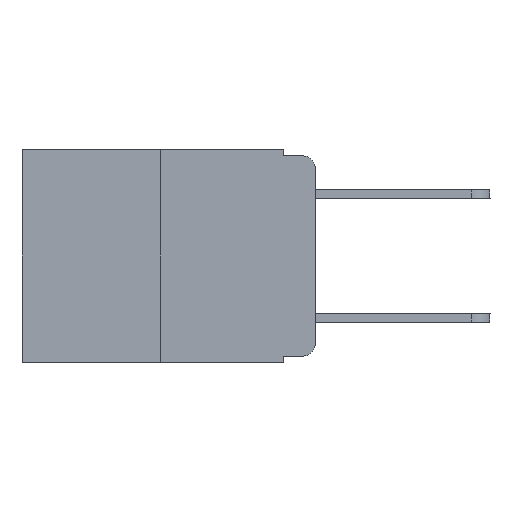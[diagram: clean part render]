
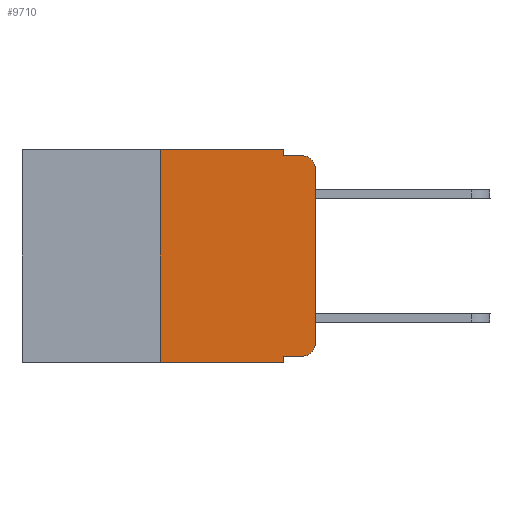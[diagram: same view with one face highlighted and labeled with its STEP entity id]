
A CAD part, left-side view. The second image highlights one B-rep face of the part: STEP entity #9710.
In plain terms, the highlighted planar face has unit normal (-1, 0, 0).
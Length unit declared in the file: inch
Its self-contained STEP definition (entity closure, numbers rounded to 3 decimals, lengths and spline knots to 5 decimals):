
#53 = CARTESIAN_POINT ( 'NONE',  ( 0., 0.02, -0.313 ) ) ;
#161 = VECTOR ( 'NONE', #4071, 39.37008 ) ;
#212 = DIRECTION ( 'NONE',  ( 1., 0., 0. ) ) ;
#253 = VECTOR ( 'NONE', #6656, 39.37008 ) ;
#276 = DIRECTION ( 'NONE',  ( 0., -1., 0. ) ) ;
#301 = ORIENTED_EDGE ( 'NONE', *, *, #6651, .F. ) ;
#363 = DIRECTION ( 'NONE',  ( 0., 0., 1. ) ) ;
#500 = CARTESIAN_POINT ( 'NONE',  ( 0., 0., 0. ) ) ;
#543 = EDGE_LOOP ( 'NONE', ( #8076, #6305, #7824, #6847, #2883, #301, #1526, #4783, #4809, #9727 ) ) ;
#1196 = EDGE_CURVE ( 'NONE', #5977, #3756, #8181, .T. ) ;
#1275 = CARTESIAN_POINT ( 'NONE',  ( 0., 0.25, -0.343 ) ) ;
#1448 = VECTOR ( 'NONE', #2631, 39.37008 ) ;
#1488 = VECTOR ( 'NONE', #363, 39.37008 ) ;
#1526 = ORIENTED_EDGE ( 'NONE', *, *, #3667, .T. ) ;
#1585 = CARTESIAN_POINT ( 'NONE',  ( 0., 0.051, -0.01 ) ) ;
#1654 = CARTESIAN_POINT ( 'NONE',  ( 0., 0.02, -0.333 ) ) ;
#1941 = VECTOR ( 'NONE', #3297, 39.37008 ) ;
#2204 = VECTOR ( 'NONE', #9762, 39.37008 ) ;
#2264 = LINE ( 'NONE', #6695, #253 ) ;
#2532 = CIRCLE ( 'NONE', #7644, 0.02 ) ;
#2631 = DIRECTION ( 'NONE',  ( 0., 0., 1. ) ) ;
#2684 = VERTEX_POINT ( 'NONE', #1654 ) ;
#2691 = CARTESIAN_POINT ( 'NONE',  ( 0., 0.02, -0.03 ) ) ;
#2705 = CARTESIAN_POINT ( 'NONE',  ( 0., 0.051, -0.01 ) ) ;
#2770 = VECTOR ( 'NONE', #276, 39.37008 ) ;
#2883 = ORIENTED_EDGE ( 'NONE', *, *, #5691, .F. ) ;
#3196 = CARTESIAN_POINT ( 'NONE',  ( 0., 0.473, -0.343 ) ) ;
#3252 = LINE ( 'NONE', #7106, #1488 ) ;
#3297 = DIRECTION ( 'NONE',  ( 0., 0., -1. ) ) ;
#3446 = VERTEX_POINT ( 'NONE', #4098 ) ;
#3496 = LINE ( 'NONE', #8485, #5391 ) ;
#3667 = EDGE_CURVE ( 'NONE', #3702, #3756, #6582, .T. ) ;
#3702 = VERTEX_POINT ( 'NONE', #1275 ) ;
#3756 = VERTEX_POINT ( 'NONE', #5948 ) ;
#3767 = VERTEX_POINT ( 'NONE', #5079 ) ;
#3789 = DIRECTION ( 'NONE',  ( 0., 0., -1. ) ) ;
#4066 = PLANE ( 'NONE',  #6803 ) ;
#4071 = DIRECTION ( 'NONE',  ( 0., -1., 0. ) ) ;
#4098 = CARTESIAN_POINT ( 'NONE',  ( 0., 0.02, -0.01 ) ) ;
#4783 = ORIENTED_EDGE ( 'NONE', *, *, #1196, .F. ) ;
#4801 = CARTESIAN_POINT ( 'NONE',  ( 0., 0.051, 0. ) ) ;
#4809 = ORIENTED_EDGE ( 'NONE', *, *, #5874, .T. ) ;
#5079 = CARTESIAN_POINT ( 'NONE',  ( 0., 0., -0.03 ) ) ;
#5333 = CARTESIAN_POINT ( 'NONE',  ( 0., 0.473, 0. ) ) ;
#5391 = VECTOR ( 'NONE', #6882, 39.37008 ) ;
#5424 = EDGE_CURVE ( 'NONE', #3767, #3446, #7389, .T. ) ;
#5447 = FACE_OUTER_BOUND ( 'NONE', #543, .T. ) ;
#5691 = EDGE_CURVE ( 'NONE', #7209, #9743, #6231, .T. ) ;
#5874 = EDGE_CURVE ( 'NONE', #5977, #2684, #3496, .T. ) ;
#5948 = CARTESIAN_POINT ( 'NONE',  ( 0., 0.051, -0.343 ) ) ;
#5977 = VERTEX_POINT ( 'NONE', #9309 ) ;
#6093 = LINE ( 'NONE', #1585, #161 ) ;
#6231 = LINE ( 'NONE', #5333, #2204 ) ;
#6305 = ORIENTED_EDGE ( 'NONE', *, *, #5424, .T. ) ;
#6357 = CARTESIAN_POINT ( 'NONE',  ( 0., 0.473, 0. ) ) ;
#6547 = LINE ( 'NONE', #500, #1448 ) ;
#6582 = LINE ( 'NONE', #3196, #2770 ) ;
#6651 = EDGE_CURVE ( 'NONE', #3702, #7209, #3252, .T. ) ;
#6656 = DIRECTION ( 'NONE',  ( 0., 0., -1. ) ) ;
#6695 = CARTESIAN_POINT ( 'NONE',  ( 0., 0.051, 0. ) ) ;
#6803 = AXIS2_PLACEMENT_3D ( 'NONE', #6357, #212, #7838 ) ;
#6847 = ORIENTED_EDGE ( 'NONE', *, *, #9526, .F. ) ;
#6882 = DIRECTION ( 'NONE',  ( 0., -1., 0. ) ) ;
#7013 = EDGE_CURVE ( 'NONE', #2684, #7725, #2532, .T. ) ;
#7106 = CARTESIAN_POINT ( 'NONE',  ( 0., 0.25, 0. ) ) ;
#7149 = AXIS2_PLACEMENT_3D ( 'NONE', #2691, #7948, #8750 ) ;
#7209 = VERTEX_POINT ( 'NONE', #8746 ) ;
#7389 = CIRCLE ( 'NONE', #7149, 0.02 ) ;
#7644 = AXIS2_PLACEMENT_3D ( 'NONE', #53, #9180, #3789 ) ;
#7677 = EDGE_CURVE ( 'NONE', #8072, #3446, #6093, .T. ) ;
#7725 = VERTEX_POINT ( 'NONE', #9167 ) ;
#7774 = CARTESIAN_POINT ( 'NONE',  ( 0., 0.051, 0. ) ) ;
#7824 = ORIENTED_EDGE ( 'NONE', *, *, #7677, .F. ) ;
#7838 = DIRECTION ( 'NONE',  ( 0., 0., -1. ) ) ;
#7948 = DIRECTION ( 'NONE',  ( -1., 0., 0. ) ) ;
#8067 = EDGE_CURVE ( 'NONE', #7725, #3767, #6547, .T. ) ;
#8072 = VERTEX_POINT ( 'NONE', #2705 ) ;
#8076 = ORIENTED_EDGE ( 'NONE', *, *, #8067, .T. ) ;
#8181 = LINE ( 'NONE', #7774, #1941 ) ;
#8485 = CARTESIAN_POINT ( 'NONE',  ( 0., 0.051, -0.333 ) ) ;
#8746 = CARTESIAN_POINT ( 'NONE',  ( 0., 0.25, 0. ) ) ;
#8750 = DIRECTION ( 'NONE',  ( 0., 0., -1. ) ) ;
#9167 = CARTESIAN_POINT ( 'NONE',  ( 0., 0., -0.313 ) ) ;
#9180 = DIRECTION ( 'NONE',  ( -1., 0., 0. ) ) ;
#9309 = CARTESIAN_POINT ( 'NONE',  ( 0., 0.051, -0.333 ) ) ;
#9526 = EDGE_CURVE ( 'NONE', #9743, #8072, #2264, .T. ) ;
#9710 = ADVANCED_FACE ( 'NONE', ( #5447 ), #4066, .F. ) ;
#9727 = ORIENTED_EDGE ( 'NONE', *, *, #7013, .T. ) ;
#9743 = VERTEX_POINT ( 'NONE', #4801 ) ;
#9762 = DIRECTION ( 'NONE',  ( 0., -1., 0. ) ) ;
